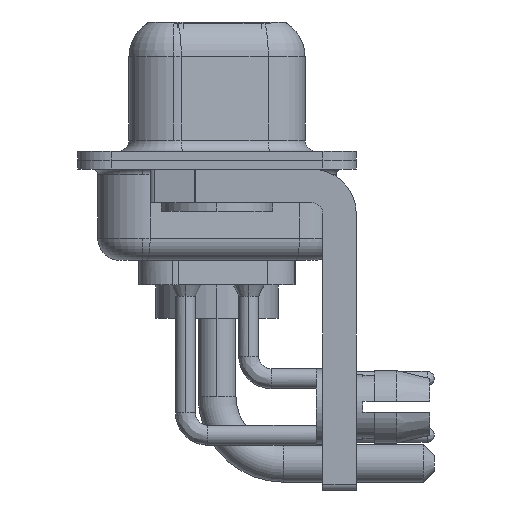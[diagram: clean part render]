
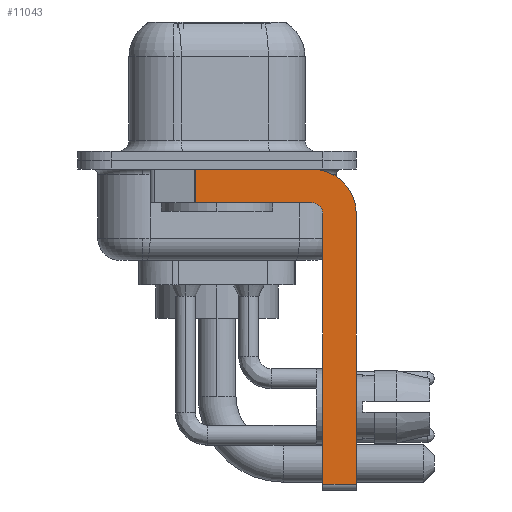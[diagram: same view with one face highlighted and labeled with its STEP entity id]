
A CAD part, left-side view. The second image highlights one B-rep face of the part: STEP entity #11043.
In plain terms, the highlighted planar face has unit normal (-1, 0, 0).
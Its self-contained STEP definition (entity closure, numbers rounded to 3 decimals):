
#224 = CARTESIAN_POINT ( 'NONE',  ( -2.9, -4.25, -2.4 ) ) ;
#335 = LINE ( 'NONE', #8530, #20092 ) ;
#461 = ORIENTED_EDGE ( 'NONE', *, *, #7290, .F. ) ;
#470 = ORIENTED_EDGE ( 'NONE', *, *, #3135, .F. ) ;
#683 = VERTEX_POINT ( 'NONE', #11030 ) ;
#1593 = VERTEX_POINT ( 'NONE', #4669 ) ;
#1987 = ORIENTED_EDGE ( 'NONE', *, *, #19664, .F. ) ;
#2606 = EDGE_CURVE ( 'NONE', #11034, #19259, #13057, .T. ) ;
#2833 = DIRECTION ( 'NONE',  ( 0., 0., 1. ) ) ;
#3135 = EDGE_CURVE ( 'NONE', #1593, #8328, #13220, .T. ) ;
#3661 = CARTESIAN_POINT ( 'NONE',  ( -2.9, -4.25, -0.4 ) ) ;
#3690 = DIRECTION ( 'NONE',  ( 0., 1., 0. ) ) ;
#3724 = DIRECTION ( 'NONE',  ( 0., 0., 1. ) ) ;
#3856 = LINE ( 'NONE', #10279, #10943 ) ;
#3929 = AXIS2_PLACEMENT_3D ( 'NONE', #15989, #12734, #2833 ) ;
#4617 = EDGE_CURVE ( 'NONE', #5609, #14761, #3856, .T. ) ;
#4669 = CARTESIAN_POINT ( 'NONE',  ( -2.9, -4.75, -14.55 ) ) ;
#4825 = EDGE_LOOP ( 'NONE', ( #6247, #19403, #461, #7145, #470, #4861, #19468, #1987 ) ) ;
#4861 = ORIENTED_EDGE ( 'NONE', *, *, #8829, .T. ) ;
#4899 = CARTESIAN_POINT ( 'NONE',  ( -2.9, -4.75, -2.4 ) ) ;
#5041 = FACE_OUTER_BOUND ( 'NONE', #4825, .T. ) ;
#5481 = DIRECTION ( 'NONE',  ( 1., 0., 0. ) ) ;
#5527 = DIRECTION ( 'NONE',  ( 0., -1., 0. ) ) ;
#5609 = VERTEX_POINT ( 'NONE', #8726 ) ;
#5865 = DIRECTION ( 'NONE',  ( 0., 0., -1. ) ) ;
#6247 = ORIENTED_EDGE ( 'NONE', *, *, #4617, .F. ) ;
#6311 = CARTESIAN_POINT ( 'NONE',  ( -2.9, -6.25, -2.4 ) ) ;
#6864 = CARTESIAN_POINT ( 'NONE',  ( -2.9, -4.75, -14.8 ) ) ;
#7079 = AXIS2_PLACEMENT_3D ( 'NONE', #14985, #5481, #20659 ) ;
#7145 = ORIENTED_EDGE ( 'NONE', *, *, #7698, .F. ) ;
#7290 = EDGE_CURVE ( 'NONE', #16466, #683, #335, .T. ) ;
#7698 = EDGE_CURVE ( 'NONE', #8328, #16466, #17050, .T. ) ;
#8103 = DIRECTION ( 'NONE',  ( 1., 0., 0. ) ) ;
#8328 = VERTEX_POINT ( 'NONE', #4899 ) ;
#8530 = CARTESIAN_POINT ( 'NONE',  ( -2.9, -4.25, -1.9 ) ) ;
#8726 = CARTESIAN_POINT ( 'NONE',  ( -2.9, 0.978, -0.4 ) ) ;
#8774 = CARTESIAN_POINT ( 'NONE',  ( -2.9, -6.25, -14.55 ) ) ;
#8829 = EDGE_CURVE ( 'NONE', #1593, #19259, #10058, .T. ) ;
#9670 = DIRECTION ( 'NONE',  ( 0., 0., -1. ) ) ;
#9845 = CARTESIAN_POINT ( 'NONE',  ( -2.9, -4.25, -14.55 ) ) ;
#10058 = LINE ( 'NONE', #9845, #15414 ) ;
#10279 = CARTESIAN_POINT ( 'NONE',  ( -2.9, 3., -0.4 ) ) ;
#10943 = VECTOR ( 'NONE', #5527, 1000. ) ;
#11030 = CARTESIAN_POINT ( 'NONE',  ( -2.9, 0.978, -1.9 ) ) ;
#11034 = VERTEX_POINT ( 'NONE', #6311 ) ;
#11043 = ADVANCED_FACE ( 'NONE', ( #5041 ), #17691, .F. ) ;
#11366 = DIRECTION ( 'NONE',  ( 0., 0., -1. ) ) ;
#11420 = EDGE_CURVE ( 'NONE', #5609, #683, #14103, .T. ) ;
#12311 = CARTESIAN_POINT ( 'NONE',  ( -2.9, -4.25, -1.9 ) ) ;
#12577 = VECTOR ( 'NONE', #3724, 1000. ) ;
#12734 = DIRECTION ( 'NONE',  ( -1., 0., 0. ) ) ;
#12965 = VECTOR ( 'NONE', #5865, 1000. ) ;
#13057 = LINE ( 'NONE', #17678, #14920 ) ;
#13220 = LINE ( 'NONE', #6864, #12577 ) ;
#14000 = CARTESIAN_POINT ( 'NONE',  ( -2.9, 0.978, -1.9 ) ) ;
#14103 = LINE ( 'NONE', #14000, #12965 ) ;
#14761 = VERTEX_POINT ( 'NONE', #3661 ) ;
#14920 = VECTOR ( 'NONE', #9670, 1000. ) ;
#14985 = CARTESIAN_POINT ( 'NONE',  ( -2.9, -4.25, -2.4 ) ) ;
#15414 = VECTOR ( 'NONE', #17756, 1000. ) ;
#15989 = CARTESIAN_POINT ( 'NONE',  ( -2.9, -4.25, -2.4 ) ) ;
#16160 = CIRCLE ( 'NONE', #7079, 2. ) ;
#16466 = VERTEX_POINT ( 'NONE', #12311 ) ;
#17050 = CIRCLE ( 'NONE', #3929, 0.5 ) ;
#17678 = CARTESIAN_POINT ( 'NONE',  ( -2.9, -6.25, -2.4 ) ) ;
#17691 = PLANE ( 'NONE',  #18831 ) ;
#17756 = DIRECTION ( 'NONE',  ( 0., -1., 0. ) ) ;
#18831 = AXIS2_PLACEMENT_3D ( 'NONE', #224, #8103, #11366 ) ;
#19259 = VERTEX_POINT ( 'NONE', #8774 ) ;
#19403 = ORIENTED_EDGE ( 'NONE', *, *, #11420, .T. ) ;
#19468 = ORIENTED_EDGE ( 'NONE', *, *, #2606, .F. ) ;
#19664 = EDGE_CURVE ( 'NONE', #14761, #11034, #16160, .T. ) ;
#20092 = VECTOR ( 'NONE', #3690, 1000. ) ;
#20659 = DIRECTION ( 'NONE',  ( 0., 0., -1. ) ) ;
